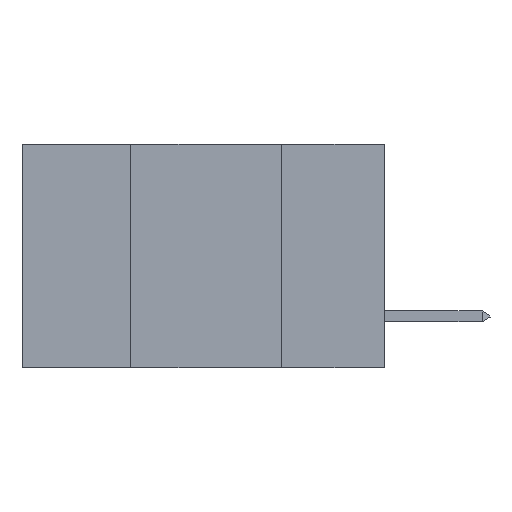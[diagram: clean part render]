
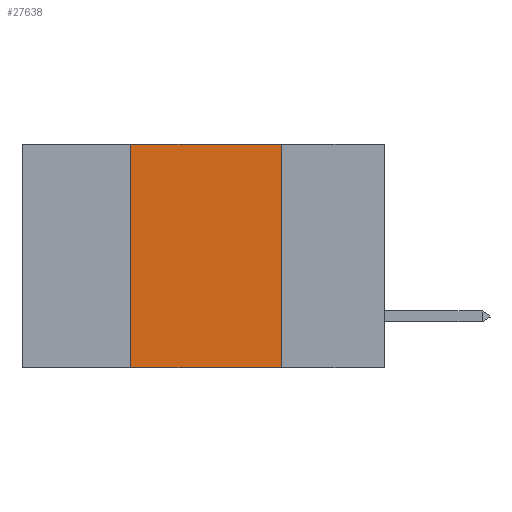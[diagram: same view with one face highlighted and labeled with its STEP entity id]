
A CAD part, left-side view. The second image highlights one B-rep face of the part: STEP entity #27638.
In plain terms, the highlighted planar face has unit normal (-1, 0, 0).
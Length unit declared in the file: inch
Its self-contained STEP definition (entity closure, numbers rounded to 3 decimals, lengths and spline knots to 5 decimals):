
#84 = VECTOR ( 'NONE', #25415, 39.37008 ) ;
#293 = EDGE_CURVE ( 'NONE', #32536, #13248, #25934, .T. ) ;
#535 = AXIS2_PLACEMENT_3D ( 'NONE', #1453, #1328, #23383 ) ;
#1207 = CARTESIAN_POINT ( 'NONE',  ( 0., 0.6, 0. ) ) ;
#1328 = DIRECTION ( 'NONE',  ( 1., 0., 0. ) ) ;
#1453 = CARTESIAN_POINT ( 'NONE',  ( 0., 0.6, 0. ) ) ;
#1693 = CARTESIAN_POINT ( 'NONE',  ( 0., 0.42, 0. ) ) ;
#3667 = CARTESIAN_POINT ( 'NONE',  ( 0., 0.42, 0. ) ) ;
#3992 = VECTOR ( 'NONE', #28887, 39.37008 ) ;
#5555 = ORIENTED_EDGE ( 'NONE', *, *, #34339, .F. ) ;
#5752 = CARTESIAN_POINT ( 'NONE',  ( 0., 0.6, -0.37 ) ) ;
#5824 = VERTEX_POINT ( 'NONE', #10350 ) ;
#6547 = CARTESIAN_POINT ( 'NONE',  ( 0., 0.42, -0.37 ) ) ;
#8716 = ORIENTED_EDGE ( 'NONE', *, *, #34293, .T. ) ;
#10082 = EDGE_CURVE ( 'NONE', #13248, #5824, #10160, .T. ) ;
#10160 = LINE ( 'NONE', #24927, #15876 ) ;
#10330 = EDGE_LOOP ( 'NONE', ( #19449, #14952, #5555, #8716 ) ) ;
#10350 = CARTESIAN_POINT ( 'NONE',  ( 0., 0.17, -0.37 ) ) ;
#12026 = CARTESIAN_POINT ( 'NONE',  ( 0., 0.17, 0. ) ) ;
#12150 = VECTOR ( 'NONE', #16940, 39.37008 ) ;
#13248 = VERTEX_POINT ( 'NONE', #12026 ) ;
#14523 = VERTEX_POINT ( 'NONE', #6547 ) ;
#14952 = ORIENTED_EDGE ( 'NONE', *, *, #293, .F. ) ;
#15876 = VECTOR ( 'NONE', #25904, 39.37008 ) ;
#16940 = DIRECTION ( 'NONE',  ( 0., 0., 1. ) ) ;
#19449 = ORIENTED_EDGE ( 'NONE', *, *, #10082, .F. ) ;
#20574 = PLANE ( 'NONE',  #535 ) ;
#23383 = DIRECTION ( 'NONE',  ( 0., 0., -1. ) ) ;
#24908 = FACE_OUTER_BOUND ( 'NONE', #10330, .T. ) ;
#24927 = CARTESIAN_POINT ( 'NONE',  ( 0., 0.17, 0. ) ) ;
#25415 = DIRECTION ( 'NONE',  ( 0., -1., 0. ) ) ;
#25904 = DIRECTION ( 'NONE',  ( 0., 0., -1. ) ) ;
#25934 = LINE ( 'NONE', #1207, #3992 ) ;
#26423 = LINE ( 'NONE', #5752, #84 ) ;
#27638 = ADVANCED_FACE ( 'NONE', ( #24908 ), #20574, .F. ) ;
#28887 = DIRECTION ( 'NONE',  ( 0., -1., 0. ) ) ;
#32536 = VERTEX_POINT ( 'NONE', #1693 ) ;
#34092 = LINE ( 'NONE', #3667, #12150 ) ;
#34293 = EDGE_CURVE ( 'NONE', #14523, #5824, #26423, .T. ) ;
#34339 = EDGE_CURVE ( 'NONE', #14523, #32536, #34092, .T. ) ;
